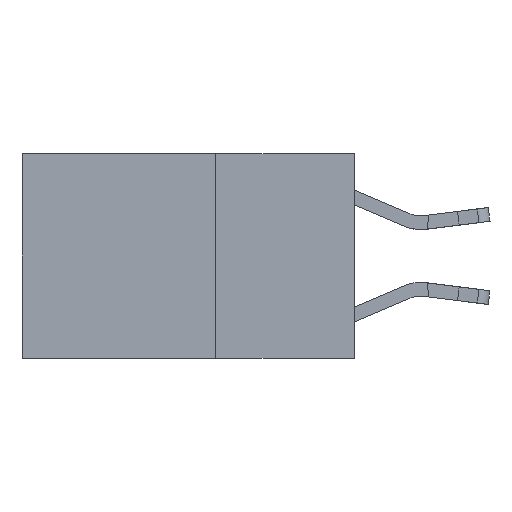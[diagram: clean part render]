
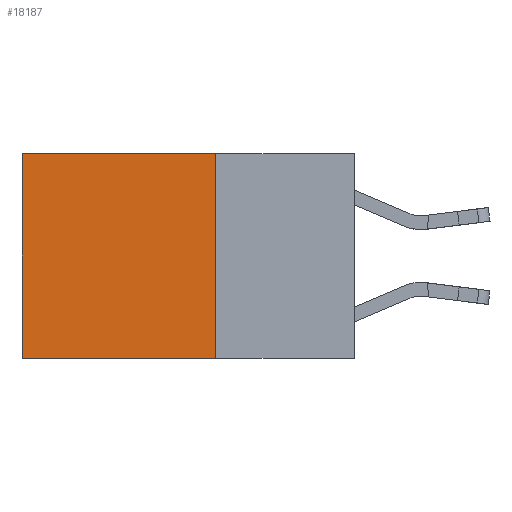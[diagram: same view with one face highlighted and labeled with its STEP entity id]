
A CAD part, left-side view. The second image highlights one B-rep face of the part: STEP entity #18187.
In plain terms, the highlighted planar face has unit normal (-1, 0, 0).
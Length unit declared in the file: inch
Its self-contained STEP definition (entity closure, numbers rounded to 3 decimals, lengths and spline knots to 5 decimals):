
#403 = CARTESIAN_POINT ( 'NONE',  ( 0.2625, 0.25, -0.37 ) ) ;
#2953 = CARTESIAN_POINT ( 'NONE',  ( 0.2625, 0.6, -0.37 ) ) ;
#3117 = EDGE_CURVE ( 'NONE', #11727, #7075, #16374, .T. ) ;
#3250 = CARTESIAN_POINT ( 'NONE',  ( 0.2625, 0.25, 0. ) ) ;
#4362 = ORIENTED_EDGE ( 'NONE', *, *, #4425, .F. ) ;
#4425 = EDGE_CURVE ( 'NONE', #10549, #14302, #21213, .T. ) ;
#4751 = EDGE_CURVE ( 'NONE', #7075, #14302, #10543, .T. ) ;
#5106 = VECTOR ( 'NONE', #12262, 39.37008 ) ;
#5766 = DIRECTION ( 'NONE',  ( 0., 0., -1. ) ) ;
#6619 = VECTOR ( 'NONE', #18975, 39.37008 ) ;
#7075 = VERTEX_POINT ( 'NONE', #20849 ) ;
#7154 = DIRECTION ( 'NONE',  ( 0., 0., -1. ) ) ;
#9370 = CARTESIAN_POINT ( 'NONE',  ( 0.2625, 0.25, 0. ) ) ;
#10404 = CARTESIAN_POINT ( 'NONE',  ( 0.2625, 0.6, 0. ) ) ;
#10543 = LINE ( 'NONE', #10404, #5106 ) ;
#10549 = VERTEX_POINT ( 'NONE', #403 ) ;
#11154 = ORIENTED_EDGE ( 'NONE', *, *, #19963, .F. ) ;
#11199 = PLANE ( 'NONE',  #16971 ) ;
#11410 = VECTOR ( 'NONE', #18393, 39.37008 ) ;
#11727 = VERTEX_POINT ( 'NONE', #3250 ) ;
#12262 = DIRECTION ( 'NONE',  ( 0., 0., -1. ) ) ;
#13673 = ORIENTED_EDGE ( 'NONE', *, *, #4751, .T. ) ;
#13725 = EDGE_LOOP ( 'NONE', ( #13673, #4362, #11154, #18624 ) ) ;
#14302 = VERTEX_POINT ( 'NONE', #2953 ) ;
#15661 = LINE ( 'NONE', #16291, #19994 ) ;
#16291 = CARTESIAN_POINT ( 'NONE',  ( 0.2625, 0.25, 0. ) ) ;
#16374 = LINE ( 'NONE', #17127, #6619 ) ;
#16531 = CARTESIAN_POINT ( 'NONE',  ( 0.2625, 0.25, -0.37 ) ) ;
#16756 = DIRECTION ( 'NONE',  ( 1., 0., 0. ) ) ;
#16971 = AXIS2_PLACEMENT_3D ( 'NONE', #9370, #16756, #5766 ) ;
#17127 = CARTESIAN_POINT ( 'NONE',  ( 0.2625, 0.25, 0. ) ) ;
#18187 = ADVANCED_FACE ( 'NONE', ( #20077 ), #11199, .F. ) ;
#18393 = DIRECTION ( 'NONE',  ( 0., 1., 0. ) ) ;
#18624 = ORIENTED_EDGE ( 'NONE', *, *, #3117, .T. ) ;
#18975 = DIRECTION ( 'NONE',  ( 0., 1., 0. ) ) ;
#19963 = EDGE_CURVE ( 'NONE', #11727, #10549, #15661, .T. ) ;
#19994 = VECTOR ( 'NONE', #7154, 39.37008 ) ;
#20077 = FACE_OUTER_BOUND ( 'NONE', #13725, .T. ) ;
#20849 = CARTESIAN_POINT ( 'NONE',  ( 0.2625, 0.6, 0. ) ) ;
#21213 = LINE ( 'NONE', #16531, #11410 ) ;
